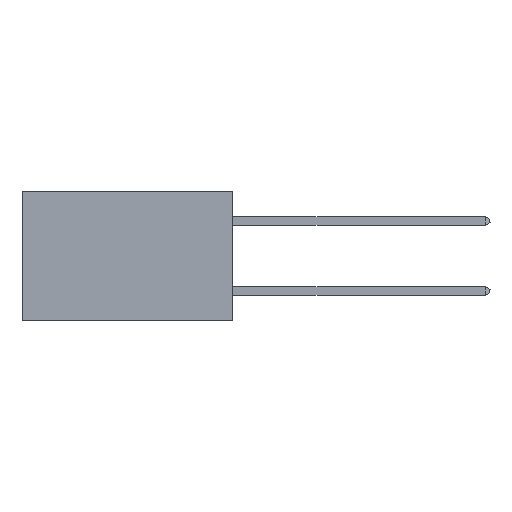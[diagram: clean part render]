
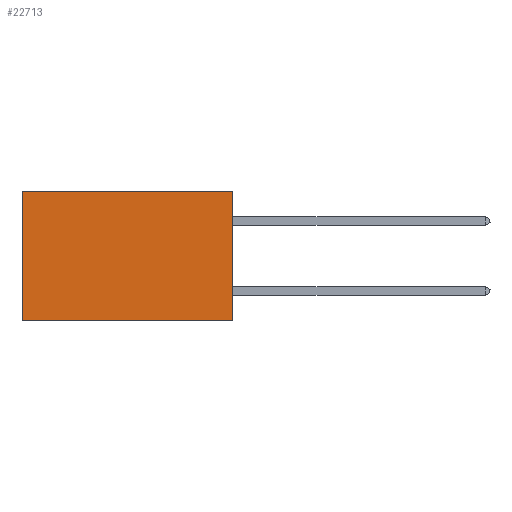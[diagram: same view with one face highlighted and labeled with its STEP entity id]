
A CAD part, left-side view. The second image highlights one B-rep face of the part: STEP entity #22713.
In plain terms, the highlighted planar face has unit normal (-1, 0, 0).
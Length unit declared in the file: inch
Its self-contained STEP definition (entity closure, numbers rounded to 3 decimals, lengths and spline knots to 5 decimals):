
#2035 = VECTOR ( 'NONE', #24162, 39.37008 ) ;
#4748 = LINE ( 'NONE', #6135, #7379 ) ;
#6135 = CARTESIAN_POINT ( 'NONE',  ( 0.2875, 0.6, 0. ) ) ;
#7019 = ORIENTED_EDGE ( 'NONE', *, *, #11333, .F. ) ;
#7379 = VECTOR ( 'NONE', #18206, 39.37008 ) ;
#9562 = VERTEX_POINT ( 'NONE', #18433 ) ;
#10451 = CARTESIAN_POINT ( 'NONE',  ( 0.2875, 0.6, 0. ) ) ;
#10647 = EDGE_CURVE ( 'NONE', #29869, #9562, #4748, .T. ) ;
#10838 = ORIENTED_EDGE ( 'NONE', *, *, #21153, .F. ) ;
#11333 = EDGE_CURVE ( 'NONE', #19668, #9562, #11523, .T. ) ;
#11523 = LINE ( 'NONE', #14396, #2035 ) ;
#11689 = AXIS2_PLACEMENT_3D ( 'NONE', #21030, #18779, #15923 ) ;
#12523 = VECTOR ( 'NONE', #29551, 39.37008 ) ;
#12822 = VECTOR ( 'NONE', #16351, 39.37008 ) ;
#12881 = CARTESIAN_POINT ( 'NONE',  ( 0.2875, 0., 0. ) ) ;
#13575 = EDGE_LOOP ( 'NONE', ( #23718, #7019, #10838, #22946 ) ) ;
#14396 = CARTESIAN_POINT ( 'NONE',  ( 0.2875, 0., -0.37 ) ) ;
#15923 = DIRECTION ( 'NONE',  ( 0., 0., -1. ) ) ;
#16351 = DIRECTION ( 'NONE',  ( 0., 0., -1. ) ) ;
#17832 = FACE_OUTER_BOUND ( 'NONE', #13575, .T. ) ;
#18206 = DIRECTION ( 'NONE',  ( 0., 0., -1. ) ) ;
#18433 = CARTESIAN_POINT ( 'NONE',  ( 0.2875, 0.6, -0.37 ) ) ;
#18688 = CARTESIAN_POINT ( 'NONE',  ( 0.2875, 0., 0. ) ) ;
#18779 = DIRECTION ( 'NONE',  ( 1., 0., 0. ) ) ;
#19668 = VERTEX_POINT ( 'NONE', #20689 ) ;
#20099 = EDGE_CURVE ( 'NONE', #27175, #29869, #22778, .T. ) ;
#20689 = CARTESIAN_POINT ( 'NONE',  ( 0.2875, 0., -0.37 ) ) ;
#21030 = CARTESIAN_POINT ( 'NONE',  ( 0.2875, 0., 0. ) ) ;
#21153 = EDGE_CURVE ( 'NONE', #27175, #19668, #22678, .T. ) ;
#22678 = LINE ( 'NONE', #18688, #12822 ) ;
#22713 = ADVANCED_FACE ( 'NONE', ( #17832 ), #23331, .F. ) ;
#22778 = LINE ( 'NONE', #12881, #12523 ) ;
#22946 = ORIENTED_EDGE ( 'NONE', *, *, #20099, .T. ) ;
#23331 = PLANE ( 'NONE',  #11689 ) ;
#23718 = ORIENTED_EDGE ( 'NONE', *, *, #10647, .T. ) ;
#24162 = DIRECTION ( 'NONE',  ( 0., 1., 0. ) ) ;
#27175 = VERTEX_POINT ( 'NONE', #29386 ) ;
#29386 = CARTESIAN_POINT ( 'NONE',  ( 0.2875, 0., 0. ) ) ;
#29551 = DIRECTION ( 'NONE',  ( 0., 1., 0. ) ) ;
#29869 = VERTEX_POINT ( 'NONE', #10451 ) ;
